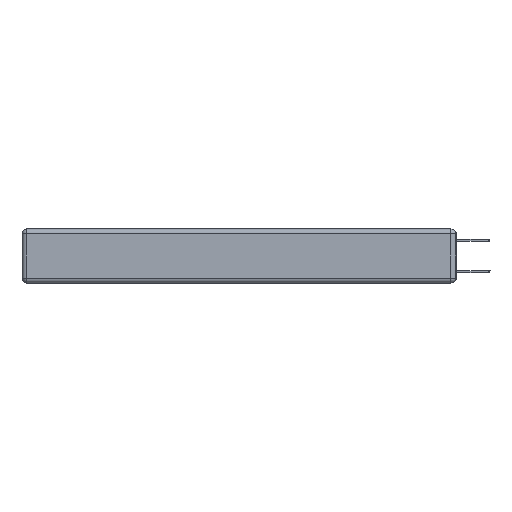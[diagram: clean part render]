
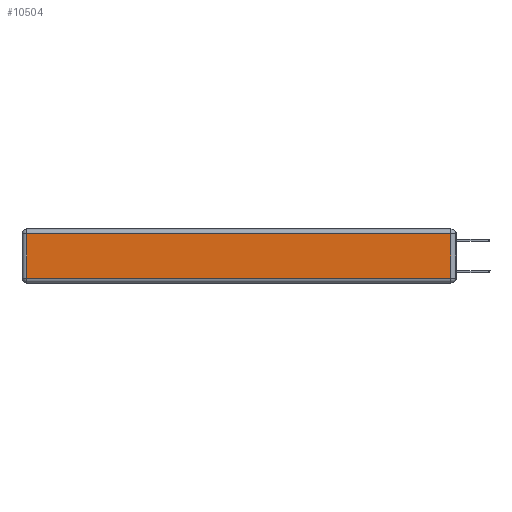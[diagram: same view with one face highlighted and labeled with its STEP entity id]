
A CAD part, left-side view. The second image highlights one B-rep face of the part: STEP entity #10504.
In plain terms, the highlighted planar face has unit normal (-1, 0, 0).
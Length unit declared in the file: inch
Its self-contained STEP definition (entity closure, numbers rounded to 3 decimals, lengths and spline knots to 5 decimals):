
#754 = CARTESIAN_POINT ( 'NONE',  ( 0., 0.03, -0.03 ) ) ;
#2517 = DIRECTION ( 'NONE',  ( 0., 0., 1. ) ) ;
#3891 = VERTEX_POINT ( 'NONE', #13891 ) ;
#4078 = VECTOR ( 'NONE', #15198, 39.37008 ) ;
#4328 = DIRECTION ( 'NONE',  ( 0., 1., 0. ) ) ;
#4740 = DIRECTION ( 'NONE',  ( 0., 0., -1. ) ) ;
#4811 = CARTESIAN_POINT ( 'NONE',  ( 0., 0.03, -0.343 ) ) ;
#5216 = ORIENTED_EDGE ( 'NONE', *, *, #6916, .T. ) ;
#6465 = DIRECTION ( 'NONE',  ( -1., 0., 0. ) ) ;
#6502 = LINE ( 'NONE', #13465, #11270 ) ;
#6806 = VECTOR ( 'NONE', #4740, 39.37008 ) ;
#6916 = EDGE_CURVE ( 'NONE', #9017, #3891, #6502, .T. ) ;
#8541 = VERTEX_POINT ( 'NONE', #14227 ) ;
#8684 = CARTESIAN_POINT ( 'NONE',  ( 0., 0., -0.313 ) ) ;
#9017 = VERTEX_POINT ( 'NONE', #754 ) ;
#9176 = CARTESIAN_POINT ( 'NONE',  ( 0., 0., -0.343 ) ) ;
#10067 = ORIENTED_EDGE ( 'NONE', *, *, #10146, .T. ) ;
#10146 = EDGE_CURVE ( 'NONE', #3891, #8541, #12409, .T. ) ;
#10307 = LINE ( 'NONE', #8684, #13380 ) ;
#10504 = ADVANCED_FACE ( 'NONE', ( #15468 ), #15752, .T. ) ;
#11270 = VECTOR ( 'NONE', #4328, 39.37008 ) ;
#11281 = CARTESIAN_POINT ( 'NONE',  ( 0., 2.72, -0.343 ) ) ;
#11609 = EDGE_CURVE ( 'NONE', #8541, #16750, #10307, .T. ) ;
#11625 = EDGE_CURVE ( 'NONE', #16750, #9017, #14414, .T. ) ;
#12409 = LINE ( 'NONE', #11281, #6806 ) ;
#13380 = VECTOR ( 'NONE', #14045, 39.37008 ) ;
#13465 = CARTESIAN_POINT ( 'NONE',  ( 0., 2.75, -0.03 ) ) ;
#13484 = ORIENTED_EDGE ( 'NONE', *, *, #11609, .T. ) ;
#13514 = AXIS2_PLACEMENT_3D ( 'NONE', #9176, #6465, #2517 ) ;
#13891 = CARTESIAN_POINT ( 'NONE',  ( 0., 2.72, -0.03 ) ) ;
#14045 = DIRECTION ( 'NONE',  ( 0., -1., 0. ) ) ;
#14227 = CARTESIAN_POINT ( 'NONE',  ( 0., 2.72, -0.313 ) ) ;
#14414 = LINE ( 'NONE', #4811, #4078 ) ;
#14674 = ORIENTED_EDGE ( 'NONE', *, *, #11625, .T. ) ;
#14719 = EDGE_LOOP ( 'NONE', ( #13484, #14674, #5216, #10067 ) ) ;
#15108 = CARTESIAN_POINT ( 'NONE',  ( 0., 0.03, -0.313 ) ) ;
#15198 = DIRECTION ( 'NONE',  ( 0., 0., 1. ) ) ;
#15468 = FACE_OUTER_BOUND ( 'NONE', #14719, .T. ) ;
#15752 = PLANE ( 'NONE',  #13514 ) ;
#16750 = VERTEX_POINT ( 'NONE', #15108 ) ;
